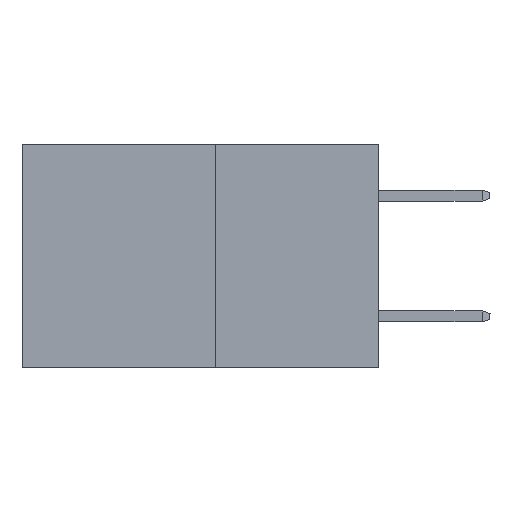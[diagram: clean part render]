
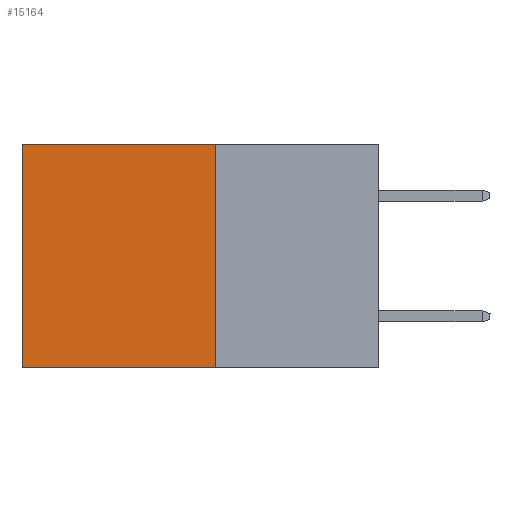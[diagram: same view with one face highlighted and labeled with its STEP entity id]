
A CAD part, left-side view. The second image highlights one B-rep face of the part: STEP entity #15164.
In plain terms, the highlighted planar face has unit normal (-1, 0, 0).
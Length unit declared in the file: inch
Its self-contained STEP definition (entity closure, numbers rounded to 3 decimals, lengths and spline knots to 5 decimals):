
#675 = CARTESIAN_POINT ( 'NONE',  ( 0.277, 0.27, 0. ) ) ;
#732 = DIRECTION ( 'NONE',  ( 1., 0., 0. ) ) ;
#1012 = EDGE_CURVE ( 'NONE', #5543, #21384, #19427, .T. ) ;
#1565 = LINE ( 'NONE', #4550, #21035 ) ;
#1657 = CARTESIAN_POINT ( 'NONE',  ( 0.277, 0.59, 0. ) ) ;
#2131 = ORIENTED_EDGE ( 'NONE', *, *, #1012, .T. ) ;
#2613 = DIRECTION ( 'NONE',  ( 0., 1., 0. ) ) ;
#2930 = CARTESIAN_POINT ( 'NONE',  ( 0.277, 0.59, -0.37 ) ) ;
#3053 = ORIENTED_EDGE ( 'NONE', *, *, #7571, .F. ) ;
#4300 = CARTESIAN_POINT ( 'NONE',  ( 0.277, 0.27, -0.37 ) ) ;
#4550 = CARTESIAN_POINT ( 'NONE',  ( 0.277, 0.27, -0.37 ) ) ;
#5325 = FACE_OUTER_BOUND ( 'NONE', #22785, .T. ) ;
#5388 = CARTESIAN_POINT ( 'NONE',  ( 0.277, 0.27, -0.37 ) ) ;
#5543 = VERTEX_POINT ( 'NONE', #1657 ) ;
#7058 = VECTOR ( 'NONE', #2613, 39.37008 ) ;
#7289 = CARTESIAN_POINT ( 'NONE',  ( 0.277, 0.27, 0. ) ) ;
#7571 = EDGE_CURVE ( 'NONE', #9915, #21384, #9731, .T. ) ;
#8526 = VECTOR ( 'NONE', #11298, 39.37008 ) ;
#8640 = PLANE ( 'NONE',  #11675 ) ;
#9215 = VECTOR ( 'NONE', #14592, 39.37008 ) ;
#9731 = LINE ( 'NONE', #5388, #8526 ) ;
#9915 = VERTEX_POINT ( 'NONE', #4300 ) ;
#10529 = DIRECTION ( 'NONE',  ( 0., 0., -1. ) ) ;
#11298 = DIRECTION ( 'NONE',  ( 0., 1., 0. ) ) ;
#11675 = AXIS2_PLACEMENT_3D ( 'NONE', #20133, #732, #14425 ) ;
#14035 = LINE ( 'NONE', #675, #7058 ) ;
#14425 = DIRECTION ( 'NONE',  ( 0., 0., -1. ) ) ;
#14592 = DIRECTION ( 'NONE',  ( 0., 0., -1. ) ) ;
#15164 = ADVANCED_FACE ( 'NONE', ( #5325 ), #8640, .F. ) ;
#15929 = ORIENTED_EDGE ( 'NONE', *, *, #16888, .F. ) ;
#16101 = VERTEX_POINT ( 'NONE', #7289 ) ;
#16576 = ORIENTED_EDGE ( 'NONE', *, *, #19617, .T. ) ;
#16888 = EDGE_CURVE ( 'NONE', #16101, #9915, #1565, .T. ) ;
#19427 = LINE ( 'NONE', #2930, #9215 ) ;
#19617 = EDGE_CURVE ( 'NONE', #16101, #5543, #14035, .T. ) ;
#20133 = CARTESIAN_POINT ( 'NONE',  ( 0.277, 0.27, -0.37 ) ) ;
#21035 = VECTOR ( 'NONE', #10529, 39.37008 ) ;
#21384 = VERTEX_POINT ( 'NONE', #24901 ) ;
#22785 = EDGE_LOOP ( 'NONE', ( #2131, #3053, #15929, #16576 ) ) ;
#24901 = CARTESIAN_POINT ( 'NONE',  ( 0.277, 0.59, -0.37 ) ) ;
